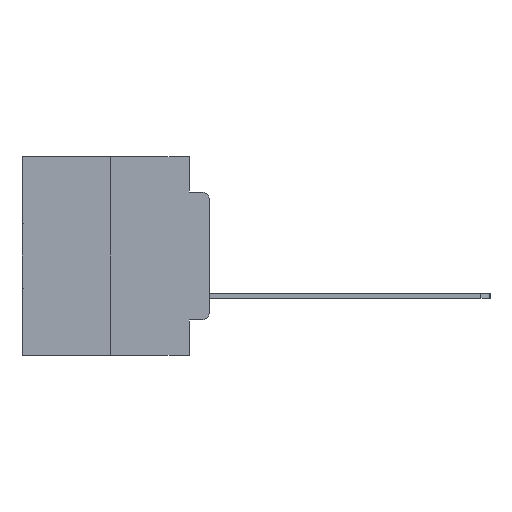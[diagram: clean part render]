
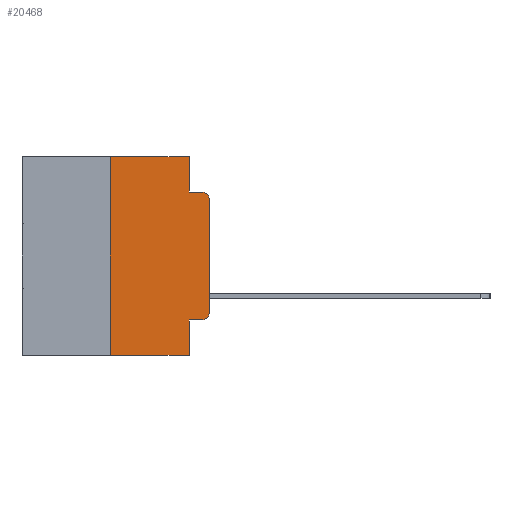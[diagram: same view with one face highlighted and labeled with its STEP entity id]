
A CAD part, left-side view. The second image highlights one B-rep face of the part: STEP entity #20468.
In plain terms, the highlighted planar face has unit normal (-1, 0, 0).
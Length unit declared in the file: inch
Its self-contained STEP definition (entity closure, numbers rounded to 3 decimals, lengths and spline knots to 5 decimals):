
#412 = DIRECTION ( 'NONE',  ( 0., -1., 0. ) ) ;
#597 = ORIENTED_EDGE ( 'NONE', *, *, #12161, .F. ) ;
#649 = VERTEX_POINT ( 'NONE', #20207 ) ;
#884 = CARTESIAN_POINT ( 'NONE',  ( 0., 0.051, 0. ) ) ;
#1597 = CARTESIAN_POINT ( 'NONE',  ( 0., 0.473, 0. ) ) ;
#2117 = EDGE_CURVE ( 'NONE', #25349, #649, #2595, .T. ) ;
#2577 = VERTEX_POINT ( 'NONE', #24249 ) ;
#2595 = LINE ( 'NONE', #7709, #11806 ) ;
#2725 = ORIENTED_EDGE ( 'NONE', *, *, #4913, .F. ) ;
#3427 = VERTEX_POINT ( 'NONE', #6356 ) ;
#3526 = VECTOR ( 'NONE', #18111, 39.37008 ) ;
#3901 = DIRECTION ( 'NONE',  ( 1., 0., 0. ) ) ;
#4361 = LINE ( 'NONE', #21894, #21504 ) ;
#4476 = ORIENTED_EDGE ( 'NONE', *, *, #7107, .T. ) ;
#4512 = VERTEX_POINT ( 'NONE', #27798 ) ;
#4854 = ORIENTED_EDGE ( 'NONE', *, *, #21140, .T. ) ;
#4913 = EDGE_CURVE ( 'NONE', #27826, #19065, #24737, .T. ) ;
#6303 = DIRECTION ( 'NONE',  ( 0., -1., 0. ) ) ;
#6307 = EDGE_CURVE ( 'NONE', #16523, #21727, #12671, .T. ) ;
#6356 = CARTESIAN_POINT ( 'NONE',  ( 0., 0.25, -0.5 ) ) ;
#6804 = DIRECTION ( 'NONE',  ( 0., 0., 1. ) ) ;
#6942 = CARTESIAN_POINT ( 'NONE',  ( 0., 0.473, -0.5 ) ) ;
#7020 = ORIENTED_EDGE ( 'NONE', *, *, #27888, .T. ) ;
#7107 = EDGE_CURVE ( 'NONE', #13723, #649, #9454, .T. ) ;
#7332 = AXIS2_PLACEMENT_3D ( 'NONE', #24533, #11316, #26727 ) ;
#7709 = CARTESIAN_POINT ( 'NONE',  ( 0., 0.051, -0.0885 ) ) ;
#7794 = VECTOR ( 'NONE', #412, 39.37008 ) ;
#8782 = VECTOR ( 'NONE', #15884, 39.37008 ) ;
#8807 = EDGE_LOOP ( 'NONE', ( #21612, #4476, #17863, #597, #2725, #14738, #4854, #28425, #7020, #24689 ) ) ;
#9454 = CIRCLE ( 'NONE', #10176, 0.02 ) ;
#9556 = LINE ( 'NONE', #22389, #3526 ) ;
#10144 = CARTESIAN_POINT ( 'NONE',  ( 0., 0.051, -0.0885 ) ) ;
#10176 = AXIS2_PLACEMENT_3D ( 'NONE', #11991, #27368, #14245 ) ;
#10438 = EDGE_CURVE ( 'NONE', #4512, #2577, #23094, .T. ) ;
#11316 = DIRECTION ( 'NONE',  ( -1., 0., 0. ) ) ;
#11690 = LINE ( 'NONE', #22316, #28512 ) ;
#11806 = VECTOR ( 'NONE', #18279, 39.37008 ) ;
#11991 = CARTESIAN_POINT ( 'NONE',  ( 0., 0.02, -0.1085 ) ) ;
#12161 = EDGE_CURVE ( 'NONE', #19065, #25349, #11690, .T. ) ;
#12172 = VECTOR ( 'NONE', #6804, 39.37008 ) ;
#12671 = CIRCLE ( 'NONE', #7332, 0.02 ) ;
#13561 = DIRECTION ( 'NONE',  ( 0., 0., -1. ) ) ;
#13723 = VERTEX_POINT ( 'NONE', #19036 ) ;
#13993 = CARTESIAN_POINT ( 'NONE',  ( 0., 0.051, 0. ) ) ;
#14245 = DIRECTION ( 'NONE',  ( 0., 0., -1. ) ) ;
#14738 = ORIENTED_EDGE ( 'NONE', *, *, #24539, .F. ) ;
#15118 = PLANE ( 'NONE',  #27238 ) ;
#15439 = LINE ( 'NONE', #6942, #8782 ) ;
#15838 = FACE_OUTER_BOUND ( 'NONE', #8807, .T. ) ;
#15884 = DIRECTION ( 'NONE',  ( 0., -1., 0. ) ) ;
#16523 = VERTEX_POINT ( 'NONE', #23874 ) ;
#16678 = DIRECTION ( 'NONE',  ( 0., 0., -1. ) ) ;
#17287 = VECTOR ( 'NONE', #16678, 39.37008 ) ;
#17863 = ORIENTED_EDGE ( 'NONE', *, *, #2117, .F. ) ;
#18093 = LINE ( 'NONE', #20167, #12172 ) ;
#18111 = DIRECTION ( 'NONE',  ( 0., 0., 1. ) ) ;
#18279 = DIRECTION ( 'NONE',  ( 0., -1., 0. ) ) ;
#19036 = CARTESIAN_POINT ( 'NONE',  ( 0., 0., -0.1085 ) ) ;
#19065 = VERTEX_POINT ( 'NONE', #13993 ) ;
#19568 = DIRECTION ( 'NONE',  ( 0., 0., -1. ) ) ;
#20167 = CARTESIAN_POINT ( 'NONE',  ( 0., 0., 0. ) ) ;
#20182 = CARTESIAN_POINT ( 'NONE',  ( 0., 0., -0.3915 ) ) ;
#20207 = CARTESIAN_POINT ( 'NONE',  ( 0., 0.02, -0.0885 ) ) ;
#20468 = ADVANCED_FACE ( 'NONE', ( #15838 ), #15118, .F. ) ;
#20638 = CARTESIAN_POINT ( 'NONE',  ( 0., 0.473, 0. ) ) ;
#21140 = EDGE_CURVE ( 'NONE', #3427, #2577, #15439, .T. ) ;
#21504 = VECTOR ( 'NONE', #6303, 39.37008 ) ;
#21612 = ORIENTED_EDGE ( 'NONE', *, *, #28021, .T. ) ;
#21727 = VERTEX_POINT ( 'NONE', #20182 ) ;
#21894 = CARTESIAN_POINT ( 'NONE',  ( 0., 0.051, -0.4115 ) ) ;
#22316 = CARTESIAN_POINT ( 'NONE',  ( 0., 0.051, 0. ) ) ;
#22389 = CARTESIAN_POINT ( 'NONE',  ( 0., 0.25, 0. ) ) ;
#23094 = LINE ( 'NONE', #884, #17287 ) ;
#23874 = CARTESIAN_POINT ( 'NONE',  ( 0., 0.02, -0.4115 ) ) ;
#24249 = CARTESIAN_POINT ( 'NONE',  ( 0., 0.051, -0.5 ) ) ;
#24533 = CARTESIAN_POINT ( 'NONE',  ( 0., 0.02, -0.3915 ) ) ;
#24539 = EDGE_CURVE ( 'NONE', #3427, #27826, #9556, .T. ) ;
#24689 = ORIENTED_EDGE ( 'NONE', *, *, #6307, .T. ) ;
#24737 = LINE ( 'NONE', #20638, #7794 ) ;
#25349 = VERTEX_POINT ( 'NONE', #10144 ) ;
#25889 = CARTESIAN_POINT ( 'NONE',  ( 0., 0.25, 0. ) ) ;
#26727 = DIRECTION ( 'NONE',  ( 0., 0., -1. ) ) ;
#27238 = AXIS2_PLACEMENT_3D ( 'NONE', #1597, #3901, #19568 ) ;
#27368 = DIRECTION ( 'NONE',  ( -1., 0., 0. ) ) ;
#27798 = CARTESIAN_POINT ( 'NONE',  ( 0., 0.051, -0.4115 ) ) ;
#27826 = VERTEX_POINT ( 'NONE', #25889 ) ;
#27888 = EDGE_CURVE ( 'NONE', #4512, #16523, #4361, .T. ) ;
#28021 = EDGE_CURVE ( 'NONE', #21727, #13723, #18093, .T. ) ;
#28425 = ORIENTED_EDGE ( 'NONE', *, *, #10438, .F. ) ;
#28512 = VECTOR ( 'NONE', #13561, 39.37008 ) ;
